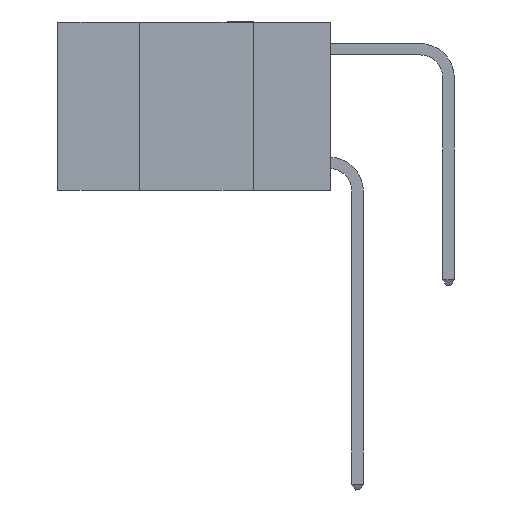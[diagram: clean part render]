
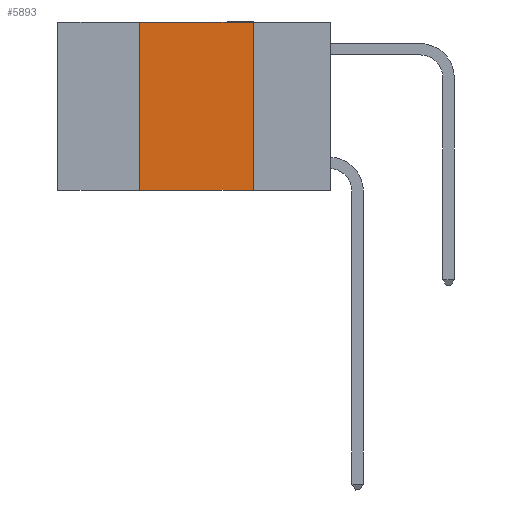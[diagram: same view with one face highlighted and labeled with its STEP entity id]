
A CAD part, left-side view. The second image highlights one B-rep face of the part: STEP entity #5893.
In plain terms, the highlighted planar face has unit normal (-1, 0, 0).
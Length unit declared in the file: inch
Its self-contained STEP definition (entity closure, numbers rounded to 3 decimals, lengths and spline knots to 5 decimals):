
#337 = EDGE_CURVE ( 'NONE', #7326, #10110, #5795, .T. ) ;
#1065 = PLANE ( 'NONE',  #7861 ) ;
#1509 = CARTESIAN_POINT ( 'NONE',  ( 0., 0.42, -0.37 ) ) ;
#2241 = EDGE_CURVE ( 'NONE', #4573, #12733, #6986, .T. ) ;
#2261 = VECTOR ( 'NONE', #12084, 39.37008 ) ;
#2412 = EDGE_CURVE ( 'NONE', #4573, #7326, #10106, .T. ) ;
#2480 = EDGE_CURVE ( 'NONE', #10110, #12733, #11783, .T. ) ;
#2770 = DIRECTION ( 'NONE',  ( 0., -1., 0. ) ) ;
#3183 = DIRECTION ( 'NONE',  ( 0., 0., -1. ) ) ;
#3296 = DIRECTION ( 'NONE',  ( 0., 0., -1. ) ) ;
#3479 = ORIENTED_EDGE ( 'NONE', *, *, #2480, .F. ) ;
#3790 = CARTESIAN_POINT ( 'NONE',  ( 0., 0.17, -0.37 ) ) ;
#4258 = CARTESIAN_POINT ( 'NONE',  ( 0., 0.17, 0. ) ) ;
#4573 = VERTEX_POINT ( 'NONE', #1509 ) ;
#5089 = DIRECTION ( 'NONE',  ( 0., -1., 0. ) ) ;
#5146 = FACE_OUTER_BOUND ( 'NONE', #5522, .T. ) ;
#5522 = EDGE_LOOP ( 'NONE', ( #3479, #8877, #11508, #9181 ) ) ;
#5774 = CARTESIAN_POINT ( 'NONE',  ( 0., 0.42, 0. ) ) ;
#5795 = LINE ( 'NONE', #12051, #8135 ) ;
#5893 = ADVANCED_FACE ( 'NONE', ( #5146 ), #1065, .F. ) ;
#6986 = LINE ( 'NONE', #10850, #11939 ) ;
#7326 = VERTEX_POINT ( 'NONE', #5774 ) ;
#7861 = AXIS2_PLACEMENT_3D ( 'NONE', #8383, #9378, #3296 ) ;
#8135 = VECTOR ( 'NONE', #5089, 39.37008 ) ;
#8383 = CARTESIAN_POINT ( 'NONE',  ( 0., 0.6, 0. ) ) ;
#8877 = ORIENTED_EDGE ( 'NONE', *, *, #337, .F. ) ;
#9146 = VECTOR ( 'NONE', #3183, 39.37008 ) ;
#9181 = ORIENTED_EDGE ( 'NONE', *, *, #2241, .T. ) ;
#9378 = DIRECTION ( 'NONE',  ( 1., 0., 0. ) ) ;
#10106 = LINE ( 'NONE', #10159, #2261 ) ;
#10110 = VERTEX_POINT ( 'NONE', #12635 ) ;
#10159 = CARTESIAN_POINT ( 'NONE',  ( 0., 0.42, 0. ) ) ;
#10850 = CARTESIAN_POINT ( 'NONE',  ( 0., 0.6, -0.37 ) ) ;
#11508 = ORIENTED_EDGE ( 'NONE', *, *, #2412, .F. ) ;
#11783 = LINE ( 'NONE', #4258, #9146 ) ;
#11939 = VECTOR ( 'NONE', #2770, 39.37008 ) ;
#12051 = CARTESIAN_POINT ( 'NONE',  ( 0., 0.6, 0. ) ) ;
#12084 = DIRECTION ( 'NONE',  ( 0., 0., 1. ) ) ;
#12635 = CARTESIAN_POINT ( 'NONE',  ( 0., 0.17, 0. ) ) ;
#12733 = VERTEX_POINT ( 'NONE', #3790 ) ;
